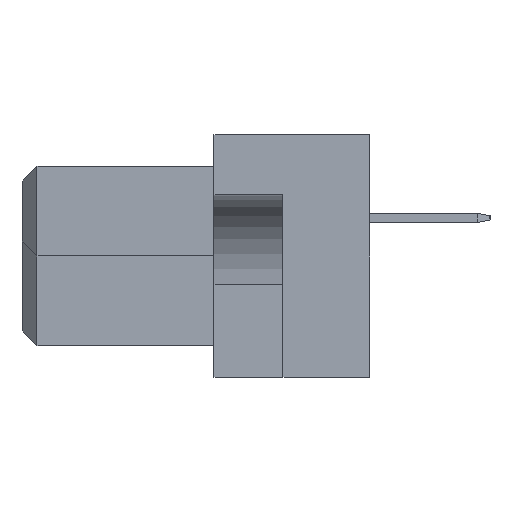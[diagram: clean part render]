
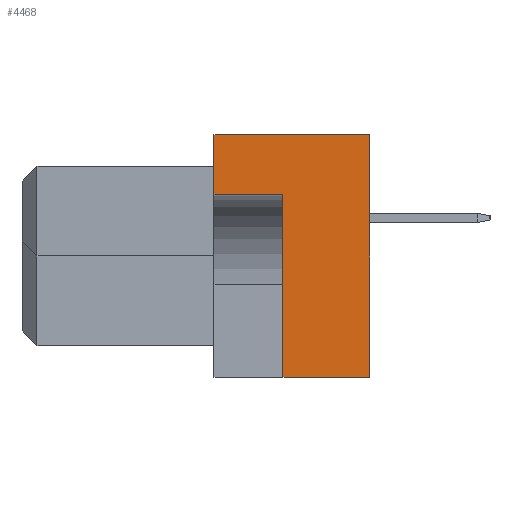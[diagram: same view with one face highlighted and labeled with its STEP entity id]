
A CAD part, left-side view. The second image highlights one B-rep face of the part: STEP entity #4468.
In plain terms, the highlighted planar face has unit normal (-1, 0, 0).
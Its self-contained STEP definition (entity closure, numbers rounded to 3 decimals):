
#507 = LINE ( 'NONE', #14789, #11555 ) ;
#509 = VERTEX_POINT ( 'NONE', #3170 ) ;
#1759 = CARTESIAN_POINT ( 'NONE',  ( -47.5, 5.2, 4.05 ) ) ;
#2045 = VECTOR ( 'NONE', #2961, 1000. ) ;
#2344 = VERTEX_POINT ( 'NONE', #17039 ) ;
#2521 = DIRECTION ( 'NONE',  ( 0., 0., 1. ) ) ;
#2792 = EDGE_CURVE ( 'NONE', #509, #4188, #21708, .T. ) ;
#2846 = LINE ( 'NONE', #17016, #22397 ) ;
#2961 = DIRECTION ( 'NONE',  ( 0., -1., 0. ) ) ;
#3170 = CARTESIAN_POINT ( 'NONE',  ( -47.5, 5.2, 2.05 ) ) ;
#3209 = DIRECTION ( 'NONE',  ( 1., 0., 0. ) ) ;
#3793 = ORIENTED_EDGE ( 'NONE', *, *, #9169, .T. ) ;
#4188 = VERTEX_POINT ( 'NONE', #1759 ) ;
#4362 = LINE ( 'NONE', #20813, #7678 ) ;
#4468 = ADVANCED_FACE ( 'NONE', ( #11577 ), #4964, .F. ) ;
#4964 = PLANE ( 'NONE',  #26150 ) ;
#4998 = VERTEX_POINT ( 'NONE', #5866 ) ;
#5745 = ORIENTED_EDGE ( 'NONE', *, *, #2792, .F. ) ;
#5866 = CARTESIAN_POINT ( 'NONE',  ( -47.5, 2.9, 2.05 ) ) ;
#7124 = CARTESIAN_POINT ( 'NONE',  ( -47.5, 5.2, 4.05 ) ) ;
#7174 = LINE ( 'NONE', #17714, #12007 ) ;
#7396 = DIRECTION ( 'NONE',  ( 0., 0., -1. ) ) ;
#7529 = ORIENTED_EDGE ( 'NONE', *, *, #11172, .F. ) ;
#7678 = VECTOR ( 'NONE', #14469, 1000. ) ;
#7995 = VECTOR ( 'NONE', #23737, 1000. ) ;
#8236 = ORIENTED_EDGE ( 'NONE', *, *, #13379, .T. ) ;
#9169 = EDGE_CURVE ( 'NONE', #16191, #24336, #507, .T. ) ;
#9441 = LINE ( 'NONE', #15364, #2045 ) ;
#10118 = EDGE_CURVE ( 'NONE', #4188, #24336, #9441, .T. ) ;
#11172 = EDGE_CURVE ( 'NONE', #2344, #4998, #4362, .T. ) ;
#11192 = CARTESIAN_POINT ( 'NONE',  ( -47.5, 5.2, 4.05 ) ) ;
#11402 = EDGE_LOOP ( 'NONE', ( #5745, #24496, #7529, #8236, #3793, #21429 ) ) ;
#11555 = VECTOR ( 'NONE', #2521, 1000. ) ;
#11577 = FACE_OUTER_BOUND ( 'NONE', #11402, .T. ) ;
#12007 = VECTOR ( 'NONE', #18822, 1000. ) ;
#13379 = EDGE_CURVE ( 'NONE', #2344, #16191, #2846, .T. ) ;
#14469 = DIRECTION ( 'NONE',  ( 0., 0., 1. ) ) ;
#14789 = CARTESIAN_POINT ( 'NONE',  ( -47.5, 0., 4.05 ) ) ;
#15119 = CARTESIAN_POINT ( 'NONE',  ( -47.5, 0., 4.05 ) ) ;
#15364 = CARTESIAN_POINT ( 'NONE',  ( -47.5, 5.2, 4.05 ) ) ;
#16191 = VERTEX_POINT ( 'NONE', #24588 ) ;
#17016 = CARTESIAN_POINT ( 'NONE',  ( -47.5, 5.2, -4.05 ) ) ;
#17039 = CARTESIAN_POINT ( 'NONE',  ( -47.5, 2.9, -4.05 ) ) ;
#17714 = CARTESIAN_POINT ( 'NONE',  ( -47.5, 2.9, 2.05 ) ) ;
#18822 = DIRECTION ( 'NONE',  ( 0., 1., 0. ) ) ;
#18934 = EDGE_CURVE ( 'NONE', #4998, #509, #7174, .T. ) ;
#20813 = CARTESIAN_POINT ( 'NONE',  ( -47.5, 2.9, 2.05 ) ) ;
#21429 = ORIENTED_EDGE ( 'NONE', *, *, #10118, .F. ) ;
#21708 = LINE ( 'NONE', #11192, #7995 ) ;
#22397 = VECTOR ( 'NONE', #25228, 1000. ) ;
#23737 = DIRECTION ( 'NONE',  ( 0., 0., 1. ) ) ;
#24336 = VERTEX_POINT ( 'NONE', #15119 ) ;
#24496 = ORIENTED_EDGE ( 'NONE', *, *, #18934, .F. ) ;
#24588 = CARTESIAN_POINT ( 'NONE',  ( -47.5, 0., -4.05 ) ) ;
#25228 = DIRECTION ( 'NONE',  ( 0., -1., 0. ) ) ;
#26150 = AXIS2_PLACEMENT_3D ( 'NONE', #7124, #3209, #7396 ) ;
